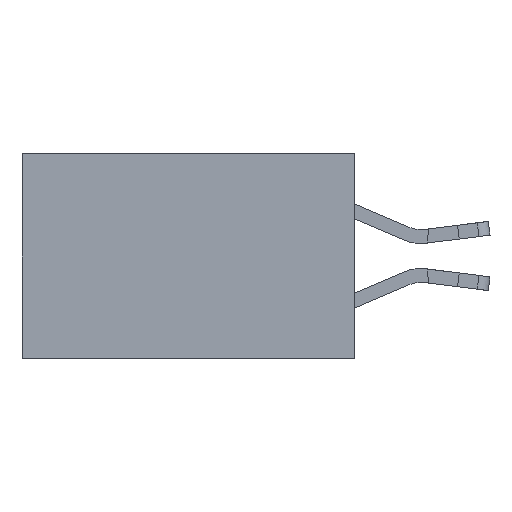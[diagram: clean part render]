
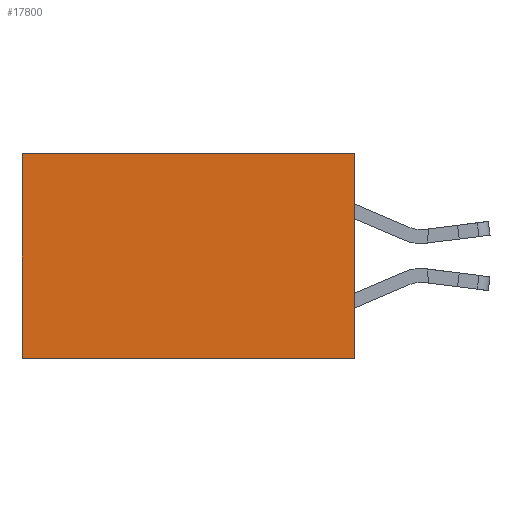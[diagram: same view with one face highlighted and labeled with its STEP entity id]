
A CAD part, left-side view. The second image highlights one B-rep face of the part: STEP entity #17800.
In plain terms, the highlighted planar face has unit normal (-1, 0, 0).
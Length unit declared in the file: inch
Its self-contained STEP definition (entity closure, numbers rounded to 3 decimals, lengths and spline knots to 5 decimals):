
#603 = DIRECTION ( 'NONE',  ( 1., 0., 0. ) ) ;
#713 = CARTESIAN_POINT ( 'NONE',  ( 0.2615, 0., -0.37 ) ) ;
#841 = VERTEX_POINT ( 'NONE', #10303 ) ;
#1092 = CARTESIAN_POINT ( 'NONE',  ( 0.2615, 0., 0. ) ) ;
#1556 = VERTEX_POINT ( 'NONE', #12254 ) ;
#1793 = CARTESIAN_POINT ( 'NONE',  ( 0.2615, 0., -0.37 ) ) ;
#2482 = DIRECTION ( 'NONE',  ( 0., 0., -1. ) ) ;
#3409 = DIRECTION ( 'NONE',  ( 0., 0., -1. ) ) ;
#3620 = EDGE_LOOP ( 'NONE', ( #9914, #12341, #7874, #5764 ) ) ;
#3917 = PLANE ( 'NONE',  #12017 ) ;
#4674 = EDGE_CURVE ( 'NONE', #1556, #11320, #6053, .T. ) ;
#4704 = VECTOR ( 'NONE', #3409, 39.37008 ) ;
#4805 = VERTEX_POINT ( 'NONE', #12864 ) ;
#5045 = LINE ( 'NONE', #9900, #11894 ) ;
#5087 = LINE ( 'NONE', #1793, #18287 ) ;
#5405 = CARTESIAN_POINT ( 'NONE',  ( 0.2615, 0.6, 0. ) ) ;
#5764 = ORIENTED_EDGE ( 'NONE', *, *, #4674, .T. ) ;
#6053 = LINE ( 'NONE', #1092, #10608 ) ;
#7874 = ORIENTED_EDGE ( 'NONE', *, *, #13466, .F. ) ;
#8081 = DIRECTION ( 'NONE',  ( 0., 1., 0. ) ) ;
#9900 = CARTESIAN_POINT ( 'NONE',  ( 0.2615, 0., -0.37 ) ) ;
#9914 = ORIENTED_EDGE ( 'NONE', *, *, #16337, .T. ) ;
#10303 = CARTESIAN_POINT ( 'NONE',  ( 0.2615, 0.6, -0.37 ) ) ;
#10608 = VECTOR ( 'NONE', #18660, 39.37008 ) ;
#11320 = VERTEX_POINT ( 'NONE', #5405 ) ;
#11888 = FACE_OUTER_BOUND ( 'NONE', #3620, .T. ) ;
#11894 = VECTOR ( 'NONE', #17759, 39.37008 ) ;
#12017 = AXIS2_PLACEMENT_3D ( 'NONE', #713, #603, #2482 ) ;
#12254 = CARTESIAN_POINT ( 'NONE',  ( 0.2615, 0., 0. ) ) ;
#12341 = ORIENTED_EDGE ( 'NONE', *, *, #18516, .F. ) ;
#12864 = CARTESIAN_POINT ( 'NONE',  ( 0.2615, 0., -0.37 ) ) ;
#13466 = EDGE_CURVE ( 'NONE', #1556, #4805, #5045, .T. ) ;
#14578 = CARTESIAN_POINT ( 'NONE',  ( 0.2615, 0.6, -0.37 ) ) ;
#16025 = LINE ( 'NONE', #14578, #4704 ) ;
#16337 = EDGE_CURVE ( 'NONE', #11320, #841, #16025, .T. ) ;
#17759 = DIRECTION ( 'NONE',  ( 0., 0., -1. ) ) ;
#17800 = ADVANCED_FACE ( 'NONE', ( #11888 ), #3917, .F. ) ;
#18287 = VECTOR ( 'NONE', #8081, 39.37008 ) ;
#18516 = EDGE_CURVE ( 'NONE', #4805, #841, #5087, .T. ) ;
#18660 = DIRECTION ( 'NONE',  ( 0., 1., 0. ) ) ;
